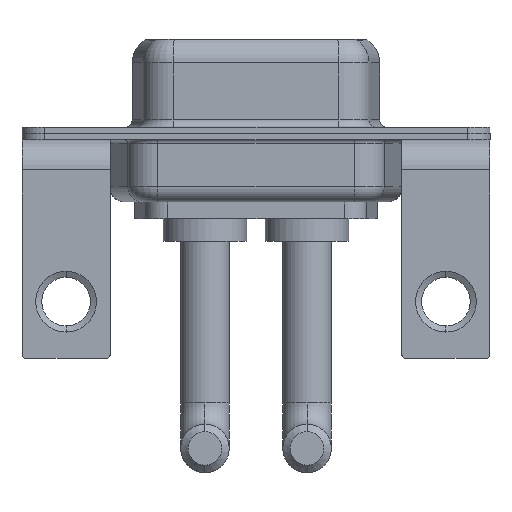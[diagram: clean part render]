
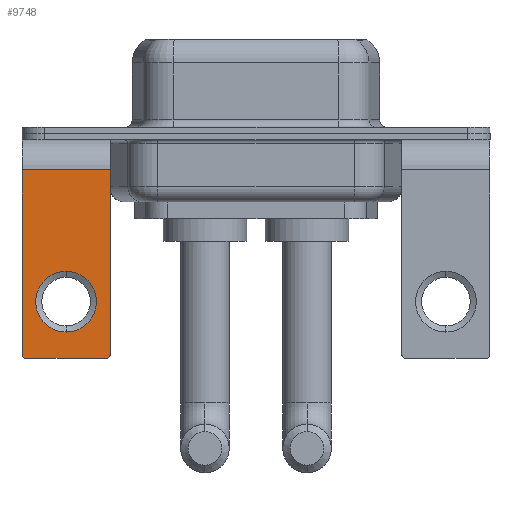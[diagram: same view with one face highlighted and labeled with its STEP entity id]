
A CAD part, front view. The second image highlights one B-rep face of the part: STEP entity #9748.
In plain terms, the highlighted planar face has unit normal (0, -1, 0).
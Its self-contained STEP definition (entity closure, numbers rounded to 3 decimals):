
#26 = VERTEX_POINT ( 'NONE', #9227 ) ;
#184 = VECTOR ( 'NONE', #11358, 1000. ) ;
#404 = CARTESIAN_POINT ( 'NONE',  ( 2.65, -6.25, -14.8 ) ) ;
#573 = DIRECTION ( 'NONE',  ( 0., 0., -1. ) ) ;
#919 = VECTOR ( 'NONE', #2029, 1000. ) ;
#1254 = CARTESIAN_POINT ( 'NONE',  ( 0., -6.25, -11.07 ) ) ;
#1264 = DIRECTION ( 'NONE',  ( 0., 1., 0. ) ) ;
#1277 = DIRECTION ( 'NONE',  ( 0., 0., 1. ) ) ;
#1288 = EDGE_CURVE ( 'NONE', #26, #6153, #4499, .T. ) ;
#1473 = CARTESIAN_POINT ( 'NONE',  ( -2.65, -6.25, -14.8 ) ) ;
#1859 = DIRECTION ( 'NONE',  ( 0., 0., 1. ) ) ;
#2029 = DIRECTION ( 'NONE',  ( 0., 0., -1. ) ) ;
#2154 = VERTEX_POINT ( 'NONE', #10036 ) ;
#2220 = EDGE_CURVE ( 'NONE', #2154, #11294, #12655, .T. ) ;
#2541 = CARTESIAN_POINT ( 'NONE',  ( -2.9, -6.25, -2.4 ) ) ;
#2664 = DIRECTION ( 'NONE',  ( -1., 0., 0. ) ) ;
#2855 = ORIENTED_EDGE ( 'NONE', *, *, #10120, .T. ) ;
#3143 = VERTEX_POINT ( 'NONE', #1473 ) ;
#3436 = VECTOR ( 'NONE', #573, 1000. ) ;
#3957 = DIRECTION ( 'NONE',  ( 0., 0., 1. ) ) ;
#4287 = LINE ( 'NONE', #10184, #184 ) ;
#4420 = ORIENTED_EDGE ( 'NONE', *, *, #11263, .T. ) ;
#4499 = LINE ( 'NONE', #2541, #3436 ) ;
#4561 = VERTEX_POINT ( 'NONE', #6209 ) ;
#4716 = CARTESIAN_POINT ( 'NONE',  ( 2.9, -6.25, -2.4 ) ) ;
#5450 = AXIS2_PLACEMENT_3D ( 'NONE', #9344, #7375, #1277 ) ;
#5488 = VERTEX_POINT ( 'NONE', #404 ) ;
#5984 = FACE_BOUND ( 'NONE', #6388, .T. ) ;
#6153 = VERTEX_POINT ( 'NONE', #7333 ) ;
#6209 = CARTESIAN_POINT ( 'NONE',  ( 2.9, -6.25, -14.55 ) ) ;
#6388 = EDGE_LOOP ( 'NONE', ( #4420, #8285 ) ) ;
#6453 = AXIS2_PLACEMENT_3D ( 'NONE', #10689, #6704, #1859 ) ;
#6606 = AXIS2_PLACEMENT_3D ( 'NONE', #1254, #12387, #11281 ) ;
#6704 = DIRECTION ( 'NONE',  ( 0., -1., 0. ) ) ;
#6779 = PLANE ( 'NONE',  #12701 ) ;
#6929 = ORIENTED_EDGE ( 'NONE', *, *, #7588, .T. ) ;
#6995 = LINE ( 'NONE', #10988, #919 ) ;
#7138 = ORIENTED_EDGE ( 'NONE', *, *, #12792, .F. ) ;
#7333 = CARTESIAN_POINT ( 'NONE',  ( -2.9, -6.25, -14.55 ) ) ;
#7375 = DIRECTION ( 'NONE',  ( 0., -1., 0. ) ) ;
#7588 = EDGE_CURVE ( 'NONE', #12044, #26, #4287, .T. ) ;
#7636 = LINE ( 'NONE', #11632, #9932 ) ;
#7752 = CIRCLE ( 'NONE', #12749, 2. ) ;
#8064 = EDGE_CURVE ( 'NONE', #5488, #4561, #11306, .T. ) ;
#8285 = ORIENTED_EDGE ( 'NONE', *, *, #2220, .T. ) ;
#9219 = EDGE_LOOP ( 'NONE', ( #12173, #2855, #7138, #9469, #11213, #6929 ) ) ;
#9227 = CARTESIAN_POINT ( 'NONE',  ( -2.9, -6.25, -2.4 ) ) ;
#9327 = CARTESIAN_POINT ( 'NONE',  ( 0., -6.25, -13.07 ) ) ;
#9344 = CARTESIAN_POINT ( 'NONE',  ( 2.65, -6.25, -14.55 ) ) ;
#9469 = ORIENTED_EDGE ( 'NONE', *, *, #8064, .T. ) ;
#9748 = ADVANCED_FACE ( 'NONE', ( #5984, #10705 ), #6779, .F. ) ;
#9932 = VECTOR ( 'NONE', #2664, 1000. ) ;
#10012 = CIRCLE ( 'NONE', #6453, 0.25 ) ;
#10036 = CARTESIAN_POINT ( 'NONE',  ( 0., -6.25, -9.07 ) ) ;
#10120 = EDGE_CURVE ( 'NONE', #6153, #3143, #10012, .T. ) ;
#10184 = CARTESIAN_POINT ( 'NONE',  ( 2.9, -6.25, -2.4 ) ) ;
#10314 = CARTESIAN_POINT ( 'NONE',  ( 0., -6.25, -11.07 ) ) ;
#10689 = CARTESIAN_POINT ( 'NONE',  ( -2.65, -6.25, -14.55 ) ) ;
#10705 = FACE_OUTER_BOUND ( 'NONE', #9219, .T. ) ;
#10988 = CARTESIAN_POINT ( 'NONE',  ( 2.9, -6.25, -2.4 ) ) ;
#11213 = ORIENTED_EDGE ( 'NONE', *, *, #12312, .F. ) ;
#11263 = EDGE_CURVE ( 'NONE', #11294, #2154, #7752, .T. ) ;
#11281 = DIRECTION ( 'NONE',  ( 0., 0., 1. ) ) ;
#11294 = VERTEX_POINT ( 'NONE', #9327 ) ;
#11306 = CIRCLE ( 'NONE', #5450, 0.25 ) ;
#11358 = DIRECTION ( 'NONE',  ( -1., 0., 0. ) ) ;
#11632 = CARTESIAN_POINT ( 'NONE',  ( 2.9, -6.25, -14.8 ) ) ;
#11759 = DIRECTION ( 'NONE',  ( 0., 1., 0. ) ) ;
#12044 = VERTEX_POINT ( 'NONE', #4716 ) ;
#12173 = ORIENTED_EDGE ( 'NONE', *, *, #1288, .T. ) ;
#12312 = EDGE_CURVE ( 'NONE', #12044, #4561, #6995, .T. ) ;
#12334 = DIRECTION ( 'NONE',  ( 0., 0., 1. ) ) ;
#12387 = DIRECTION ( 'NONE',  ( 0., 1., 0. ) ) ;
#12655 = CIRCLE ( 'NONE', #6606, 2. ) ;
#12701 = AXIS2_PLACEMENT_3D ( 'NONE', #12914, #11759, #3957 ) ;
#12749 = AXIS2_PLACEMENT_3D ( 'NONE', #10314, #1264, #12334 ) ;
#12792 = EDGE_CURVE ( 'NONE', #5488, #3143, #7636, .T. ) ;
#12914 = CARTESIAN_POINT ( 'NONE',  ( 2.9, -6.25, -2.4 ) ) ;
